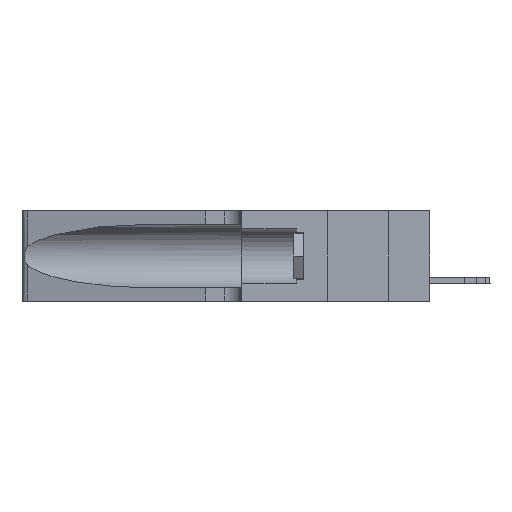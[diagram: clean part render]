
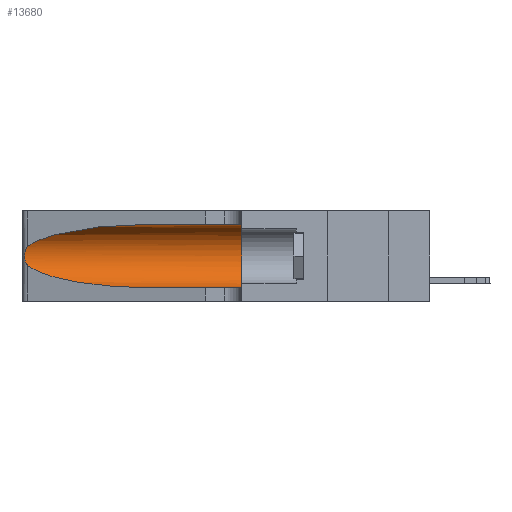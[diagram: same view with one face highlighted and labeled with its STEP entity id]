
A CAD part, left-side view. The second image highlights one B-rep face of the part: STEP entity #13680.
In plain terms, the highlighted cylindrical face has radius 3.308 mm (diameter 6.617 mm), a partial arc.
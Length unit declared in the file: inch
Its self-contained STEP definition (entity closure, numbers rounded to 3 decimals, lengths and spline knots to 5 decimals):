
#498 = CARTESIAN_POINT ( 'NONE',  ( 0.2373, 1.15595, 0.08982 ) ) ;
#1039 = VERTEX_POINT ( 'NONE', #4747 ) ;
#1292 = EDGE_CURVE ( 'NONE', #1039, #29703, #27854, .T. ) ;
#1495 = CARTESIAN_POINT ( 'NONE',  ( 0.25487, 1.22718, 0.22369 ) ) ;
#1737 = CARTESIAN_POINT ( 'NONE',  ( 0.25854, 1.2359, 0.20912 ) ) ;
#1844 = DIRECTION ( 'NONE',  ( 0., 1., 0. ) ) ;
#2108 = AXIS2_PLACEMENT_3D ( 'NONE', #3477, #1844, #23737 ) ;
#3477 = CARTESIAN_POINT ( 'NONE',  ( 0.1305, 0.35, 0.185 ) ) ;
#4034 = CARTESIAN_POINT ( 'NONE',  ( 0.1305, 0.72297, 0.05475 ) ) ;
#4747 = CARTESIAN_POINT ( 'NONE',  ( 0.1305, 0.72297, 0.31525 ) ) ;
#4835 =( BOUNDED_CURVE ( )  B_SPLINE_CURVE ( 3, ( #9779, #31776, #28681, #15550 ),
 .UNSPECIFIED., .F., .F. ) 
 B_SPLINE_CURVE_WITH_KNOTS ( ( 4, 4 ),
 ( 1.5708, 2.84003 ),
 .UNSPECIFIED. ) 
 CURVE ( )  GEOMETRIC_REPRESENTATION_ITEM ( )  RATIONAL_B_SPLINE_CURVE ( ( 1., 0.87, 0.87, 1. ) ) 
 REPRESENTATION_ITEM ( '' )  );
#5886 = B_SPLINE_CURVE_WITH_KNOTS ( 'NONE', 3,
 ( #1495, #17966, #28361, #7195, #1737, #15195, #9679, #23277, #14707, #20446, #17842, #28583, #23051, #12127 ),
 .UNSPECIFIED., .F., .F.,
 ( 4, 2, 2, 2, 2, 2, 4 ),
 ( 0., 0.00027, 0.00053, 0.00107, 0.0016, 0.00187, 0.00214 ),
 .UNSPECIFIED. ) ;
#6995 = DIRECTION ( 'NONE',  ( 0., 0., -1. ) ) ;
#7195 = CARTESIAN_POINT ( 'NONE',  ( 0.25787, 1.23484, 0.2124 ) ) ;
#7310 = DIRECTION ( 'NONE',  ( 0., -1., 0. ) ) ;
#8054 = EDGE_CURVE ( 'NONE', #29703, #25987, #21804, .T. ) ;
#8089 = ORIENTED_EDGE ( 'NONE', *, *, #8103, .T. ) ;
#8103 = EDGE_CURVE ( 'NONE', #1039, #22972, #4835, .T. ) ;
#8679 = EDGE_LOOP ( 'NONE', ( #8089, #12320, #16516, #32694, #30146, #32450 ) ) ;
#8976 = VERTEX_POINT ( 'NONE', #4034 ) ;
#9421 = VECTOR ( 'NONE', #23353, 39.37008 ) ;
#9679 = CARTESIAN_POINT ( 'NONE',  ( 0.26075, 1.23896, 0.19203 ) ) ;
#9779 = CARTESIAN_POINT ( 'NONE',  ( 0.1305, 0.72297, 0.31525 ) ) ;
#11411 = CARTESIAN_POINT ( 'NONE',  ( 0.18966, 0.96281, 0.05475 ) ) ;
#12127 = CARTESIAN_POINT ( 'NONE',  ( 0.25487, 1.22718, 0.14631 ) ) ;
#12320 = ORIENTED_EDGE ( 'NONE', *, *, #21219, .T. ) ;
#12490 = CARTESIAN_POINT ( 'NONE',  ( 0.1305, 1.61858, 0.31525 ) ) ;
#13075 =( BOUNDED_CURVE ( )  B_SPLINE_CURVE ( 3, ( #30109, #498, #11411, #19462 ),
 .UNSPECIFIED., .F., .F. ) 
 B_SPLINE_CURVE_WITH_KNOTS ( ( 4, 4 ),
 ( 3.44316, 4.71239 ),
 .UNSPECIFIED. ) 
 CURVE ( )  GEOMETRIC_REPRESENTATION_ITEM ( )  RATIONAL_B_SPLINE_CURVE ( ( 1., 0.87, 0.87, 1. ) ) 
 REPRESENTATION_ITEM ( '' )  );
#13544 = EDGE_CURVE ( 'NONE', #8976, #25987, #33062, .T. ) ;
#13680 = ADVANCED_FACE ( 'NONE', ( #24207 ), #16991, .F. ) ;
#14707 = CARTESIAN_POINT ( 'NONE',  ( 0.26017, 1.23833, 0.17102 ) ) ;
#15126 = CARTESIAN_POINT ( 'NONE',  ( 0.25487, 1.22718, 0.14631 ) ) ;
#15195 = CARTESIAN_POINT ( 'NONE',  ( 0.26018, 1.23835, 0.19895 ) ) ;
#15550 = CARTESIAN_POINT ( 'NONE',  ( 0.25487, 1.22718, 0.22369 ) ) ;
#16011 = VECTOR ( 'NONE', #7310, 39.37008 ) ;
#16516 = ORIENTED_EDGE ( 'NONE', *, *, #28968, .T. ) ;
#16991 = CYLINDRICAL_SURFACE ( 'NONE', #29856, 0.13025 ) ;
#17842 = CARTESIAN_POINT ( 'NONE',  ( 0.25789, 1.23486, 0.15765 ) ) ;
#17966 = CARTESIAN_POINT ( 'NONE',  ( 0.25555, 1.22994, 0.2215 ) ) ;
#19462 = CARTESIAN_POINT ( 'NONE',  ( 0.1305, 0.72297, 0.05475 ) ) ;
#20446 = CARTESIAN_POINT ( 'NONE',  ( 0.25856, 1.23593, 0.16098 ) ) ;
#21219 = EDGE_CURVE ( 'NONE', #22972, #21927, #5886, .T. ) ;
#21804 = CIRCLE ( 'NONE', #2108, 0.13025 ) ;
#21927 = VERTEX_POINT ( 'NONE', #15126 ) ;
#22019 = CARTESIAN_POINT ( 'NONE',  ( 0.1305, 0.35, 0.05475 ) ) ;
#22972 = VERTEX_POINT ( 'NONE', #28013 ) ;
#23051 = CARTESIAN_POINT ( 'NONE',  ( 0.25555, 1.22993, 0.14849 ) ) ;
#23277 = CARTESIAN_POINT ( 'NONE',  ( 0.26075, 1.23896, 0.178 ) ) ;
#23353 = DIRECTION ( 'NONE',  ( 0., -1., 0. ) ) ;
#23737 = DIRECTION ( 'NONE',  ( 0., 0., 1. ) ) ;
#24207 = FACE_OUTER_BOUND ( 'NONE', #8679, .T. ) ;
#25987 = VERTEX_POINT ( 'NONE', #22019 ) ;
#27854 = LINE ( 'NONE', #12490, #16011 ) ;
#28013 = CARTESIAN_POINT ( 'NONE',  ( 0.25487, 1.22718, 0.22369 ) ) ;
#28361 = CARTESIAN_POINT ( 'NONE',  ( 0.25639, 1.23184, 0.21858 ) ) ;
#28583 = CARTESIAN_POINT ( 'NONE',  ( 0.25639, 1.23186, 0.15144 ) ) ;
#28681 = CARTESIAN_POINT ( 'NONE',  ( 0.2373, 1.15595, 0.28018 ) ) ;
#28968 = EDGE_CURVE ( 'NONE', #21927, #8976, #13075, .T. ) ;
#29703 = VERTEX_POINT ( 'NONE', #34247 ) ;
#29856 = AXIS2_PLACEMENT_3D ( 'NONE', #31009, #33703, #6995 ) ;
#30109 = CARTESIAN_POINT ( 'NONE',  ( 0.25487, 1.22718, 0.14631 ) ) ;
#30146 = ORIENTED_EDGE ( 'NONE', *, *, #8054, .F. ) ;
#31009 = CARTESIAN_POINT ( 'NONE',  ( 0.1305, 1.61858, 0.185 ) ) ;
#31776 = CARTESIAN_POINT ( 'NONE',  ( 0.18966, 0.96281, 0.31525 ) ) ;
#32450 = ORIENTED_EDGE ( 'NONE', *, *, #1292, .F. ) ;
#32694 = ORIENTED_EDGE ( 'NONE', *, *, #13544, .T. ) ;
#33062 = LINE ( 'NONE', #33860, #9421 ) ;
#33703 = DIRECTION ( 'NONE',  ( 0., -1., 0. ) ) ;
#33860 = CARTESIAN_POINT ( 'NONE',  ( 0.1305, 1.61858, 0.05475 ) ) ;
#34247 = CARTESIAN_POINT ( 'NONE',  ( 0.1305, 0.35, 0.31525 ) ) ;
